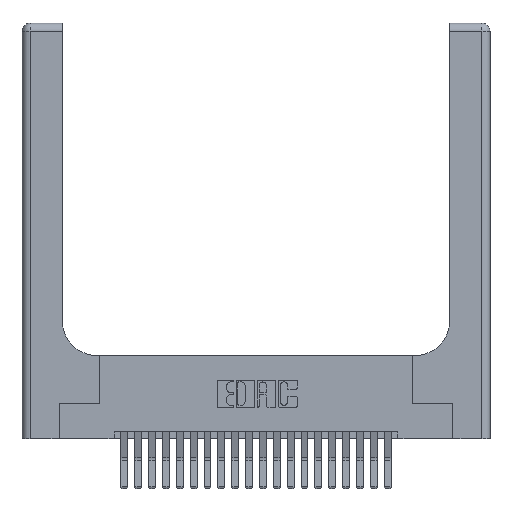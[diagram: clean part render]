
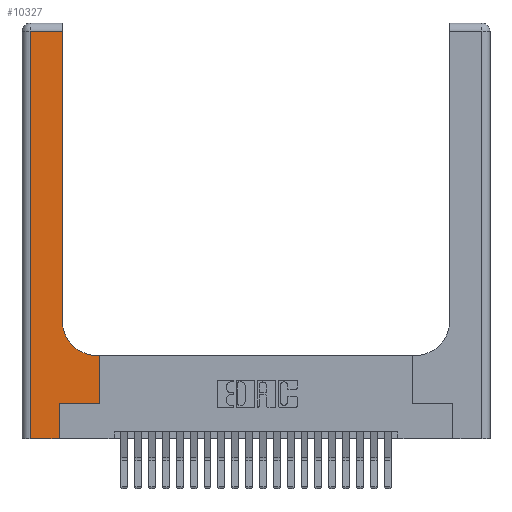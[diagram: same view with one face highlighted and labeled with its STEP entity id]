
A CAD part, top view. The second image highlights one B-rep face of the part: STEP entity #10327.
In plain terms, the highlighted planar face has unit normal (0, 0, 1).
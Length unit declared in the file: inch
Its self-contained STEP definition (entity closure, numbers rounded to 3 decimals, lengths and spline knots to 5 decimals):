
#485 = CARTESIAN_POINT ( 'NONE',  ( 0.06, 2.94, 0.37 ) ) ;
#501 = DIRECTION ( 'NONE',  ( 0., 0., -1. ) ) ;
#576 = CARTESIAN_POINT ( 'NONE',  ( 0.5415, 0.6, 0.37 ) ) ;
#673 = EDGE_CURVE ( 'NONE', #8280, #7315, #16051, .T. ) ;
#1125 = VECTOR ( 'NONE', #20924, 39.37008 ) ;
#1534 = VECTOR ( 'NONE', #20600, 39.37008 ) ;
#2366 = CARTESIAN_POINT ( 'NONE',  ( 0.5585, 0.25, 0.37 ) ) ;
#2400 = LINE ( 'NONE', #11307, #21442 ) ;
#2494 = DIRECTION ( 'NONE',  ( 1., 0., 0. ) ) ;
#2706 = CARTESIAN_POINT ( 'NONE',  ( 0.269, 0., 0.37 ) ) ;
#2821 = CARTESIAN_POINT ( 'NONE',  ( 0., 2.94, 0.37 ) ) ;
#3383 = FACE_OUTER_BOUND ( 'NONE', #8086, .T. ) ;
#3696 = CARTESIAN_POINT ( 'NONE',  ( 0.269, 0.25, 0.37 ) ) ;
#3777 = LINE ( 'NONE', #17714, #22193 ) ;
#3790 = ORIENTED_EDGE ( 'NONE', *, *, #21234, .T. ) ;
#3953 = ORIENTED_EDGE ( 'NONE', *, *, #15777, .T. ) ;
#3976 = VECTOR ( 'NONE', #17180, 39.37008 ) ;
#4311 = VERTEX_POINT ( 'NONE', #17923 ) ;
#4362 = ORIENTED_EDGE ( 'NONE', *, *, #11346, .T. ) ;
#4750 = ORIENTED_EDGE ( 'NONE', *, *, #17660, .T. ) ;
#4950 = VECTOR ( 'NONE', #19465, 39.37008 ) ;
#5198 = ORIENTED_EDGE ( 'NONE', *, *, #673, .T. ) ;
#5354 = ORIENTED_EDGE ( 'NONE', *, *, #12152, .T. ) ;
#6201 = DIRECTION ( 'NONE',  ( 0., 1., 0. ) ) ;
#6247 = PLANE ( 'NONE',  #19008 ) ;
#6882 = LINE ( 'NONE', #22696, #9480 ) ;
#6977 = VERTEX_POINT ( 'NONE', #485 ) ;
#7315 = VERTEX_POINT ( 'NONE', #3696 ) ;
#7531 = EDGE_CURVE ( 'NONE', #12941, #4311, #11031, .T. ) ;
#7667 = ORIENTED_EDGE ( 'NONE', *, *, #7531, .T. ) ;
#7790 = ORIENTED_EDGE ( 'NONE', *, *, #10278, .T. ) ;
#7832 = CARTESIAN_POINT ( 'NONE',  ( 0.06, 3., 0.37 ) ) ;
#7924 = ORIENTED_EDGE ( 'NONE', *, *, #19238, .T. ) ;
#8026 = CARTESIAN_POINT ( 'NONE',  ( 0.2915, 0.6, 0.37 ) ) ;
#8086 = EDGE_LOOP ( 'NONE', ( #3790, #3953, #4362, #4750, #5198, #5354, #7667, #7790, #7924 ) ) ;
#8110 = CARTESIAN_POINT ( 'NONE',  ( 0., 3., 0.37 ) ) ;
#8280 = VERTEX_POINT ( 'NONE', #10163 ) ;
#9480 = VECTOR ( 'NONE', #2494, 39.37008 ) ;
#9613 = CARTESIAN_POINT ( 'NONE',  ( 0.06, 0., 0.37 ) ) ;
#9991 = DIRECTION ( 'NONE',  ( 0., 0., -1. ) ) ;
#10163 = CARTESIAN_POINT ( 'NONE',  ( 0.269, 0., 0.37 ) ) ;
#10278 = EDGE_CURVE ( 'NONE', #4311, #22030, #19279, .T. ) ;
#10327 = ADVANCED_FACE ( 'NONE', ( #3383 ), #6247, .F. ) ;
#10981 = CARTESIAN_POINT ( 'NONE',  ( 0.5585, 0.25, 0.37 ) ) ;
#11031 = LINE ( 'NONE', #2366, #20115 ) ;
#11307 = CARTESIAN_POINT ( 'NONE',  ( 0.2915, 3., 0.37 ) ) ;
#11346 = EDGE_CURVE ( 'NONE', #6977, #12470, #15838, .T. ) ;
#11842 = CARTESIAN_POINT ( 'NONE',  ( 0.5415, 0.85, 0.37 ) ) ;
#12152 = EDGE_CURVE ( 'NONE', #7315, #12941, #6882, .T. ) ;
#12375 = VERTEX_POINT ( 'NONE', #14754 ) ;
#12470 = VERTEX_POINT ( 'NONE', #9613 ) ;
#12941 = VERTEX_POINT ( 'NONE', #10981 ) ;
#13668 = DIRECTION ( 'NONE',  ( 1., 0., 0. ) ) ;
#13669 = LINE ( 'NONE', #2821, #4950 ) ;
#14754 = CARTESIAN_POINT ( 'NONE',  ( 0.2915, 0.85, 0.37 ) ) ;
#15777 = EDGE_CURVE ( 'NONE', #23382, #6977, #13669, .T. ) ;
#15838 = LINE ( 'NONE', #7832, #1534 ) ;
#16051 = LINE ( 'NONE', #2706, #1125 ) ;
#17180 = DIRECTION ( 'NONE',  ( -1., 0., 0. ) ) ;
#17429 = AXIS2_PLACEMENT_3D ( 'NONE', #11842, #501, #13668 ) ;
#17660 = EDGE_CURVE ( 'NONE', #12470, #8280, #3777, .T. ) ;
#17714 = CARTESIAN_POINT ( 'NONE',  ( 0., 0., 0.37 ) ) ;
#17923 = CARTESIAN_POINT ( 'NONE',  ( 0.5585, 0.6, 0.37 ) ) ;
#19008 = AXIS2_PLACEMENT_3D ( 'NONE', #8110, #9991, #22688 ) ;
#19238 = EDGE_CURVE ( 'NONE', #22030, #12375, #22946, .T. ) ;
#19279 = LINE ( 'NONE', #8026, #3976 ) ;
#19456 = DIRECTION ( 'NONE',  ( 1., 0., 0. ) ) ;
#19465 = DIRECTION ( 'NONE',  ( -1., 0., 0. ) ) ;
#20115 = VECTOR ( 'NONE', #6201, 39.37008 ) ;
#20422 = DIRECTION ( 'NONE',  ( 0., 1., 0. ) ) ;
#20600 = DIRECTION ( 'NONE',  ( 0., -1., 0. ) ) ;
#20924 = DIRECTION ( 'NONE',  ( 0., 1., 0. ) ) ;
#21234 = EDGE_CURVE ( 'NONE', #12375, #23382, #2400, .T. ) ;
#21442 = VECTOR ( 'NONE', #20422, 39.37008 ) ;
#22030 = VERTEX_POINT ( 'NONE', #576 ) ;
#22193 = VECTOR ( 'NONE', #19456, 39.37008 ) ;
#22688 = DIRECTION ( 'NONE',  ( -1., 0., 0. ) ) ;
#22696 = CARTESIAN_POINT ( 'NONE',  ( 0.269, 0.25, 0.37 ) ) ;
#22946 = CIRCLE ( 'NONE', #17429, 0.25 ) ;
#23072 = CARTESIAN_POINT ( 'NONE',  ( 0.2915, 2.94, 0.37 ) ) ;
#23382 = VERTEX_POINT ( 'NONE', #23072 ) ;
